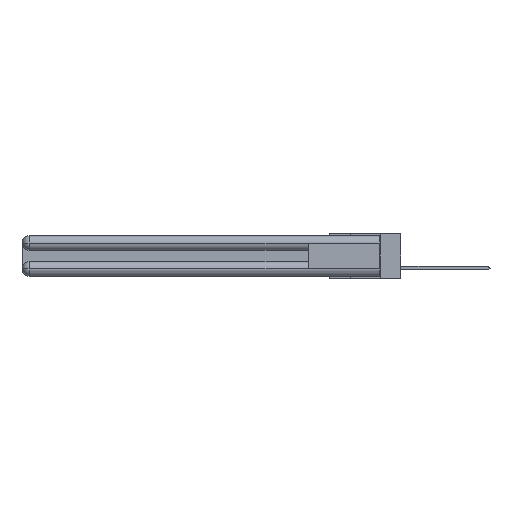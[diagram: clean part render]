
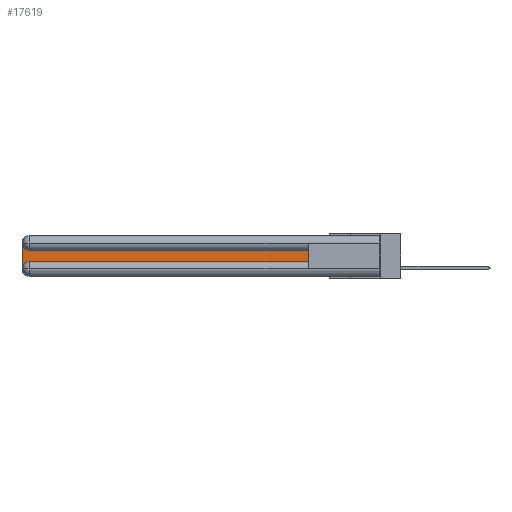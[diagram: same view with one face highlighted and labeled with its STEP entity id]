
A CAD part, left-side view. The second image highlights one B-rep face of the part: STEP entity #17619.
In plain terms, the highlighted planar face has unit normal (-1, 0, 0).
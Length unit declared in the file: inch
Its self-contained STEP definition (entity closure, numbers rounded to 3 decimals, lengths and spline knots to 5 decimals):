
#1027 = CARTESIAN_POINT ( 'NONE',  ( 0.075, 0.6, -0.1225 ) ) ;
#1569 = LINE ( 'NONE', #30033, #1951 ) ;
#1702 = AXIS2_PLACEMENT_3D ( 'NONE', #2966, #16399, #31296 ) ;
#1951 = VECTOR ( 'NONE', #3565, 39.37008 ) ;
#2360 = ORIENTED_EDGE ( 'NONE', *, *, #8041, .T. ) ;
#2522 = VECTOR ( 'NONE', #18581, 39.37008 ) ;
#2966 = CARTESIAN_POINT ( 'NONE',  ( 0.075, 2.94, -0.2775 ) ) ;
#3523 = VERTEX_POINT ( 'NONE', #4723 ) ;
#3565 = DIRECTION ( 'NONE',  ( 0., 1., 0. ) ) ;
#4008 = ORIENTED_EDGE ( 'NONE', *, *, #28908, .T. ) ;
#4585 = ORIENTED_EDGE ( 'NONE', *, *, #19550, .T. ) ;
#4723 = CARTESIAN_POINT ( 'NONE',  ( 0.075, 3., -0.2775 ) ) ;
#5861 = CARTESIAN_POINT ( 'NONE',  ( 0.075, 2.94, -0.2175 ) ) ;
#6239 = CARTESIAN_POINT ( 'NONE',  ( 0.075, 0.6, -0.2175 ) ) ;
#8041 = EDGE_CURVE ( 'NONE', #16682, #13152, #26109, .T. ) ;
#9653 = EDGE_CURVE ( 'NONE', #13152, #16678, #28266, .T. ) ;
#10112 = CARTESIAN_POINT ( 'NONE',  ( 0.075, 2.94, -0.0625 ) ) ;
#10808 = CIRCLE ( 'NONE', #1702, 0.06 ) ;
#11086 = DIRECTION ( 'NONE',  ( 0., 0., -1. ) ) ;
#11819 = DIRECTION ( 'NONE',  ( 1., 0., 0. ) ) ;
#12908 = DIRECTION ( 'NONE',  ( 0., 0., -1. ) ) ;
#13152 = VERTEX_POINT ( 'NONE', #26165 ) ;
#13806 = ORIENTED_EDGE ( 'NONE', *, *, #14393, .T. ) ;
#14393 = EDGE_CURVE ( 'NONE', #18921, #29475, #19093, .T. ) ;
#14745 = EDGE_LOOP ( 'NONE', ( #27946, #13806, #4008, #4585, #2360, #23217 ) ) ;
#16399 = DIRECTION ( 'NONE',  ( 1., 0., 0. ) ) ;
#16678 = VERTEX_POINT ( 'NONE', #1027 ) ;
#16682 = VERTEX_POINT ( 'NONE', #5861 ) ;
#17253 = CARTESIAN_POINT ( 'NONE',  ( 0.075, 2.94, -0.1225 ) ) ;
#17619 = ADVANCED_FACE ( 'NONE', ( #20758 ), #17685, .F. ) ;
#17685 = PLANE ( 'NONE',  #21704 ) ;
#17979 = VECTOR ( 'NONE', #11086, 39.37008 ) ;
#18581 = DIRECTION ( 'NONE',  ( 0., 0., 1. ) ) ;
#18921 = VERTEX_POINT ( 'NONE', #17253 ) ;
#18958 = VECTOR ( 'NONE', #19783, 39.37008 ) ;
#19093 = CIRCLE ( 'NONE', #28138, 0.06 ) ;
#19550 = EDGE_CURVE ( 'NONE', #3523, #16682, #10808, .T. ) ;
#19783 = DIRECTION ( 'NONE',  ( 0., -1., 0. ) ) ;
#20025 = CARTESIAN_POINT ( 'NONE',  ( 0.075, 3., -0.1225 ) ) ;
#20252 = LINE ( 'NONE', #20747, #17979 ) ;
#20747 = CARTESIAN_POINT ( 'NONE',  ( 0.075, 3., -0.2175 ) ) ;
#20758 = FACE_OUTER_BOUND ( 'NONE', #14745, .T. ) ;
#21704 = AXIS2_PLACEMENT_3D ( 'NONE', #20025, #25283, #12908 ) ;
#22289 = EDGE_CURVE ( 'NONE', #16678, #18921, #1569, .T. ) ;
#22939 = CARTESIAN_POINT ( 'NONE',  ( 0.075, 3., -0.0625 ) ) ;
#23217 = ORIENTED_EDGE ( 'NONE', *, *, #9653, .T. ) ;
#25283 = DIRECTION ( 'NONE',  ( 1., 0., 0. ) ) ;
#26109 = LINE ( 'NONE', #29383, #18958 ) ;
#26165 = CARTESIAN_POINT ( 'NONE',  ( 0.075, 0.6, -0.2175 ) ) ;
#27946 = ORIENTED_EDGE ( 'NONE', *, *, #22289, .T. ) ;
#28138 = AXIS2_PLACEMENT_3D ( 'NONE', #10112, #11819, #28771 ) ;
#28266 = LINE ( 'NONE', #6239, #2522 ) ;
#28771 = DIRECTION ( 'NONE',  ( 0., 0., -1. ) ) ;
#28908 = EDGE_CURVE ( 'NONE', #29475, #3523, #20252, .T. ) ;
#29383 = CARTESIAN_POINT ( 'NONE',  ( 0.075, 0.6, -0.2175 ) ) ;
#29475 = VERTEX_POINT ( 'NONE', #22939 ) ;
#30033 = CARTESIAN_POINT ( 'NONE',  ( 0.075, 0.6, -0.1225 ) ) ;
#31296 = DIRECTION ( 'NONE',  ( 0., 0., -1. ) ) ;
